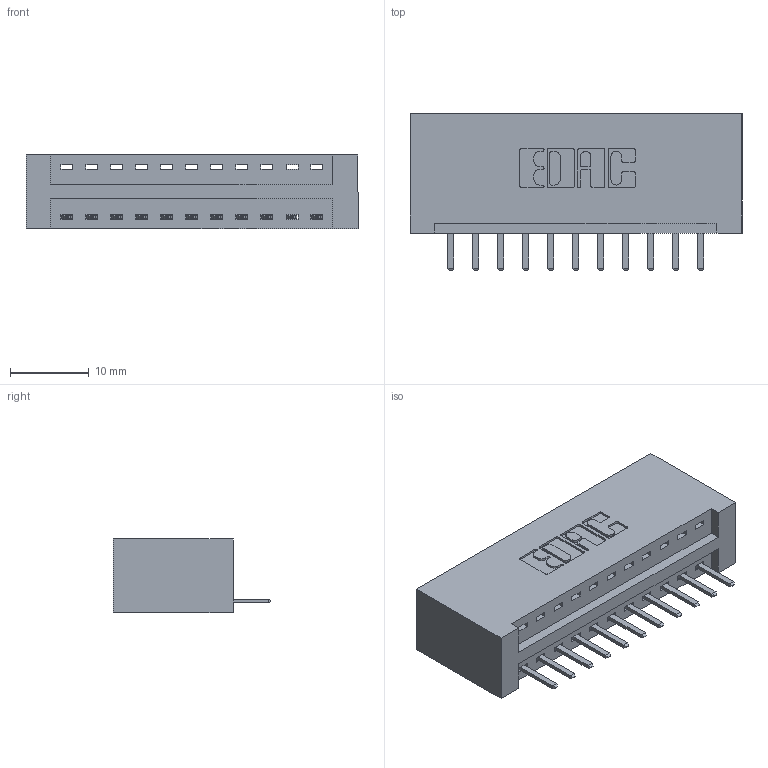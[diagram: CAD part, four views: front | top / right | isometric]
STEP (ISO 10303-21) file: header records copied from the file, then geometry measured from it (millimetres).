
FILE_DESCRIPTION (( 'STEP AP203' ), '1' );
FILE_NAME ('396-011-520-101.STEP', '2018-08-31T04:14:10', ( '' ), ( '' ), 'SwSTEP 2.0', 'SolidWorks 2016', '' );
FILE_SCHEMA (( 'CONFIG_CONTROL_DESIGN' ));
Length unit declared in the file: inch
Products named in the file (3): 346 Part_No Mounting Lugs; 345-292-001_345-293-120; 396-011-520-101
Assembly tree (12 placements, depth 2):
  396-011-520-101
    346 Part_No Mounting Lugs
    345-292-001_345-293-120  x11
Bounding box: 42.16 x 20.02 x 9.4 mm (x, y, z)
Volume: 4340.2 mm3; surface area: 5059.7 mm2
Topology: 12 solids, 12 shells, 796 faces, 2329 edges, 1522 vertices
Faces by surface type: plane 534, cylinder 262
Entity records: 10837 total; most frequent: CARTESIAN_POINT 1885, ORIENTED_EDGE 1818, DIRECTION 1683, EDGE_CURVE 909, VECTOR 737, LINE 737, VERTEX_POINT 602, AXIS2_PLACEMENT_3D 473
